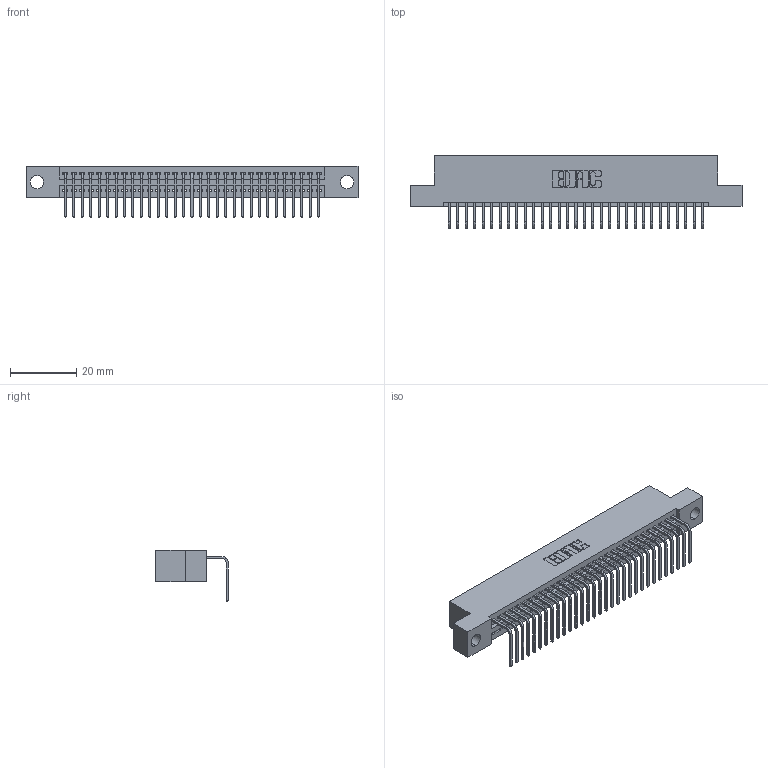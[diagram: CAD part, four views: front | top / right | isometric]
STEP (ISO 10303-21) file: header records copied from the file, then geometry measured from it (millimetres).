
FILE_DESCRIPTION (( 'STEP AP203' ), '1' );
FILE_NAME ('395-031-558-104.STEP', '2021-06-11T14:31:24', ( '' ), ( '' ), 'SwSTEP 2.0', 'SolidWorks 2020', '' );
FILE_SCHEMA (( 'CONFIG_CONTROL_DESIGN' ));
Length unit declared in the file: inch
Products named in the file (3): 345 Part_Flush Mounting Lugs - 0.156 Dia-TI; 395-031-558-104; 345-292-001_558 Tail - 2
Assembly tree (32 placements, depth 2):
  395-031-558-104
    345 Part_Flush Mounting Lugs - 0.156 Dia-TI
    345-292-001_558 Tail - 2  x31
Bounding box: 99.95 x 21.83 x 15.37 mm (x, y, z)
Volume: 9400.5 mm3; surface area: 12792.3 mm2
Topology: 32 solids, 32 shells, 2000 faces, 6019 edges, 3970 vertices
Faces by surface type: plane 1396, cylinder 604
Entity records: 25315 total; most frequent: CARTESIAN_POINT 4395, ORIENTED_EDGE 4358, DIRECTION 3853, EDGE_CURVE 2179, VECTOR 1923, LINE 1923, VERTEX_POINT 1450, AXIS2_PLACEMENT_3D 965
